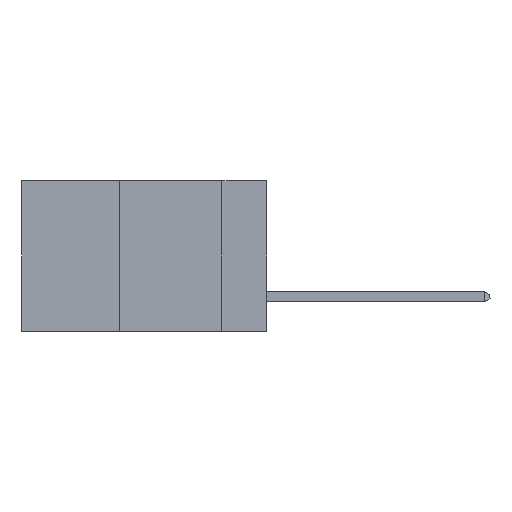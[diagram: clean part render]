
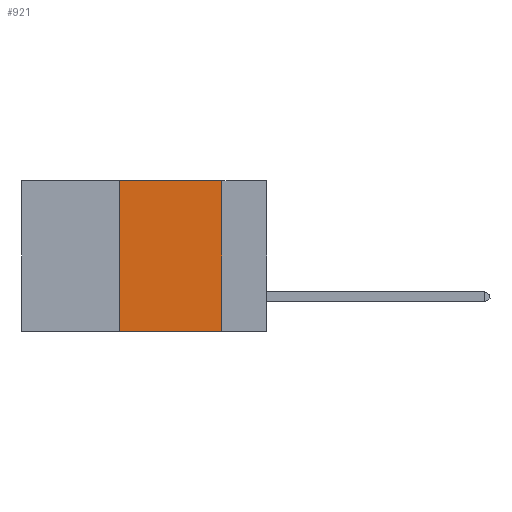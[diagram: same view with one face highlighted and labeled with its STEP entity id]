
A CAD part, left-side view. The second image highlights one B-rep face of the part: STEP entity #921.
In plain terms, the highlighted planar face has unit normal (-1, 0, 0).
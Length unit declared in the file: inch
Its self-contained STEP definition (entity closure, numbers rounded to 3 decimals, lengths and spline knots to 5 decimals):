
#827 = ORIENTED_EDGE ( 'NONE', *, *, #1844, .F. ) ;
#921 = ADVANCED_FACE ( 'NONE', ( #15842 ), #28726, .F. ) ;
#998 = VERTEX_POINT ( 'NONE', #8874 ) ;
#1224 = VECTOR ( 'NONE', #2741, 39.37008 ) ;
#1648 = ORIENTED_EDGE ( 'NONE', *, *, #24671, .T. ) ;
#1844 = EDGE_CURVE ( 'NONE', #22903, #10449, #21662, .T. ) ;
#2741 = DIRECTION ( 'NONE',  ( 0., -1., 0. ) ) ;
#3084 = LINE ( 'NONE', #34178, #31951 ) ;
#5826 = VECTOR ( 'NONE', #7774, 39.37008 ) ;
#6278 = VECTOR ( 'NONE', #30035, 39.37008 ) ;
#7038 = ORIENTED_EDGE ( 'NONE', *, *, #18786, .F. ) ;
#7200 = VERTEX_POINT ( 'NONE', #14062 ) ;
#7774 = DIRECTION ( 'NONE',  ( 0., 0., 1. ) ) ;
#8874 = CARTESIAN_POINT ( 'NONE',  ( 0., 0.36, -0.37 ) ) ;
#10449 = VERTEX_POINT ( 'NONE', #22665 ) ;
#11524 = EDGE_CURVE ( 'NONE', #998, #7200, #12622, .T. ) ;
#12622 = LINE ( 'NONE', #16366, #5826 ) ;
#14062 = CARTESIAN_POINT ( 'NONE',  ( 0., 0.36, 0. ) ) ;
#14326 = DIRECTION ( 'NONE',  ( 1., 0., 0. ) ) ;
#15842 = FACE_OUTER_BOUND ( 'NONE', #28500, .T. ) ;
#16366 = CARTESIAN_POINT ( 'NONE',  ( 0., 0.36, 0. ) ) ;
#18615 = AXIS2_PLACEMENT_3D ( 'NONE', #31598, #14326, #34419 ) ;
#18786 = EDGE_CURVE ( 'NONE', #7200, #22903, #3084, .T. ) ;
#19876 = DIRECTION ( 'NONE',  ( 0., -1., 0. ) ) ;
#20049 = CARTESIAN_POINT ( 'NONE',  ( 0., 0.6, -0.37 ) ) ;
#21349 = CARTESIAN_POINT ( 'NONE',  ( 0., 0.11, 0. ) ) ;
#21662 = LINE ( 'NONE', #21349, #6278 ) ;
#22665 = CARTESIAN_POINT ( 'NONE',  ( 0., 0.11, -0.37 ) ) ;
#22903 = VERTEX_POINT ( 'NONE', #29559 ) ;
#24671 = EDGE_CURVE ( 'NONE', #998, #10449, #30125, .T. ) ;
#28500 = EDGE_LOOP ( 'NONE', ( #827, #7038, #36603, #1648 ) ) ;
#28726 = PLANE ( 'NONE',  #18615 ) ;
#29559 = CARTESIAN_POINT ( 'NONE',  ( 0., 0.11, 0. ) ) ;
#30035 = DIRECTION ( 'NONE',  ( 0., 0., -1. ) ) ;
#30125 = LINE ( 'NONE', #20049, #1224 ) ;
#31598 = CARTESIAN_POINT ( 'NONE',  ( 0., 0.6, 0. ) ) ;
#31951 = VECTOR ( 'NONE', #19876, 39.37008 ) ;
#34178 = CARTESIAN_POINT ( 'NONE',  ( 0., 0.6, 0. ) ) ;
#34419 = DIRECTION ( 'NONE',  ( 0., 0., -1. ) ) ;
#36603 = ORIENTED_EDGE ( 'NONE', *, *, #11524, .F. ) ;
